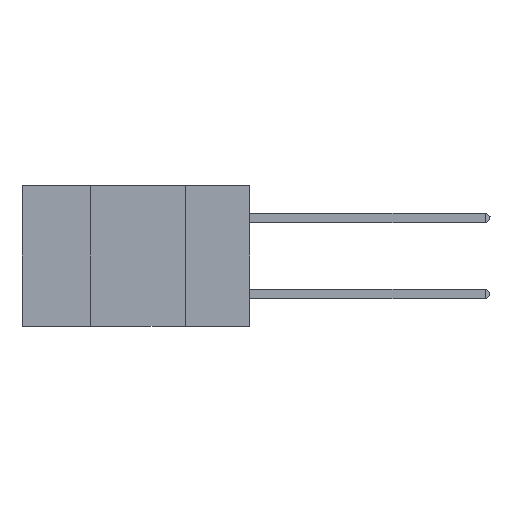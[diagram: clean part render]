
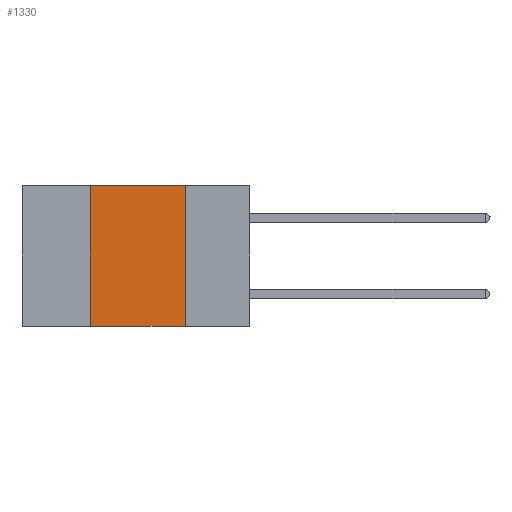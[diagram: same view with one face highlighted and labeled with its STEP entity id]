
A CAD part, left-side view. The second image highlights one B-rep face of the part: STEP entity #1330.
In plain terms, the highlighted planar face has unit normal (-1, 0, 0).
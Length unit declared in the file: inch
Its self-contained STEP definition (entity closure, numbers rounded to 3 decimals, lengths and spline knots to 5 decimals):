
#508 = CARTESIAN_POINT ( 'NONE',  ( 0., 0.6, -0.37 ) ) ;
#800 = VECTOR ( 'NONE', #7211, 39.37008 ) ;
#875 = ORIENTED_EDGE ( 'NONE', *, *, #8237, .F. ) ;
#1077 = LINE ( 'NONE', #7224, #800 ) ;
#1110 = VECTOR ( 'NONE', #3911, 39.37008 ) ;
#1330 = ADVANCED_FACE ( 'NONE', ( #7945 ), #8192, .F. ) ;
#1529 = EDGE_LOOP ( 'NONE', ( #7134, #5921, #875, #7602 ) ) ;
#2110 = VERTEX_POINT ( 'NONE', #5147 ) ;
#2387 = CARTESIAN_POINT ( 'NONE',  ( 0., 0.42, -0.37 ) ) ;
#3883 = DIRECTION ( 'NONE',  ( 0., 0., 1. ) ) ;
#3911 = DIRECTION ( 'NONE',  ( 0., -1., 0. ) ) ;
#4747 = VECTOR ( 'NONE', #6595, 39.37008 ) ;
#5147 = CARTESIAN_POINT ( 'NONE',  ( 0., 0.17, -0.37 ) ) ;
#5231 = VERTEX_POINT ( 'NONE', #6107 ) ;
#5472 = CARTESIAN_POINT ( 'NONE',  ( 0., 0.17, 0. ) ) ;
#5542 = EDGE_CURVE ( 'NONE', #5231, #7154, #1077, .T. ) ;
#5809 = CARTESIAN_POINT ( 'NONE',  ( 0., 0.17, 0. ) ) ;
#5921 = ORIENTED_EDGE ( 'NONE', *, *, #5542, .F. ) ;
#6107 = CARTESIAN_POINT ( 'NONE',  ( 0., 0.42, 0. ) ) ;
#6243 = VECTOR ( 'NONE', #3883, 39.37008 ) ;
#6595 = DIRECTION ( 'NONE',  ( 0., 0., -1. ) ) ;
#6855 = LINE ( 'NONE', #5809, #4747 ) ;
#7001 = AXIS2_PLACEMENT_3D ( 'NONE', #9683, #9681, #9534 ) ;
#7134 = ORIENTED_EDGE ( 'NONE', *, *, #9193, .F. ) ;
#7154 = VERTEX_POINT ( 'NONE', #5472 ) ;
#7201 = EDGE_CURVE ( 'NONE', #9087, #2110, #7673, .T. ) ;
#7211 = DIRECTION ( 'NONE',  ( 0., -1., 0. ) ) ;
#7224 = CARTESIAN_POINT ( 'NONE',  ( 0., 0.6, 0. ) ) ;
#7602 = ORIENTED_EDGE ( 'NONE', *, *, #7201, .T. ) ;
#7673 = LINE ( 'NONE', #508, #1110 ) ;
#7945 = FACE_OUTER_BOUND ( 'NONE', #1529, .T. ) ;
#8192 = PLANE ( 'NONE',  #7001 ) ;
#8237 = EDGE_CURVE ( 'NONE', #9087, #5231, #8338, .T. ) ;
#8338 = LINE ( 'NONE', #10059, #6243 ) ;
#9087 = VERTEX_POINT ( 'NONE', #2387 ) ;
#9193 = EDGE_CURVE ( 'NONE', #7154, #2110, #6855, .T. ) ;
#9534 = DIRECTION ( 'NONE',  ( 0., 0., -1. ) ) ;
#9681 = DIRECTION ( 'NONE',  ( 1., 0., 0. ) ) ;
#9683 = CARTESIAN_POINT ( 'NONE',  ( 0., 0.6, 0. ) ) ;
#10059 = CARTESIAN_POINT ( 'NONE',  ( 0., 0.42, 0. ) ) ;
